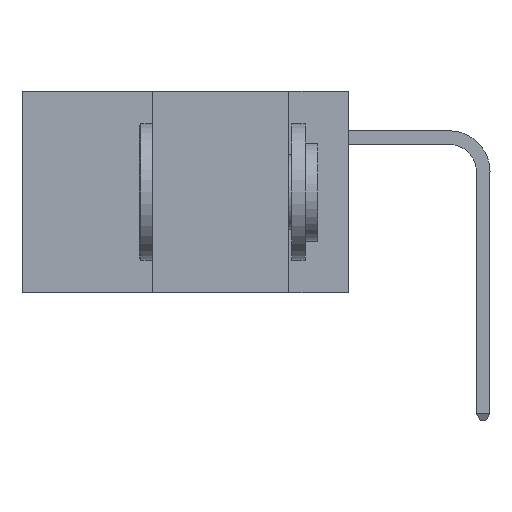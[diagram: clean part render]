
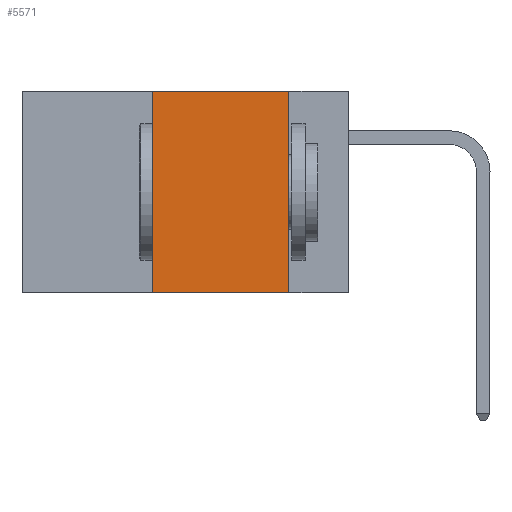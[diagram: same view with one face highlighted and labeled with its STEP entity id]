
A CAD part, left-side view. The second image highlights one B-rep face of the part: STEP entity #5571.
In plain terms, the highlighted planar face has unit normal (-1, 0, 0).
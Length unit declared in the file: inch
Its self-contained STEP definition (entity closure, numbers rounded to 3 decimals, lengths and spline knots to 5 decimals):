
#237 = CARTESIAN_POINT ( 'NONE',  ( 0., 0.36, -0.37 ) ) ;
#370 = DIRECTION ( 'NONE',  ( 0., 0., -1. ) ) ;
#1208 = AXIS2_PLACEMENT_3D ( 'NONE', #5564, #13552, #370 ) ;
#1296 = EDGE_CURVE ( 'NONE', #7038, #14603, #11462, .T. ) ;
#1375 = CARTESIAN_POINT ( 'NONE',  ( 0., 0.6, 0. ) ) ;
#2028 = LINE ( 'NONE', #10373, #7548 ) ;
#2738 = LINE ( 'NONE', #5368, #11712 ) ;
#2787 = EDGE_CURVE ( 'NONE', #7378, #13815, #3717, .T. ) ;
#3147 = EDGE_CURVE ( 'NONE', #13815, #14603, #2028, .T. ) ;
#3717 = LINE ( 'NONE', #1375, #15862 ) ;
#4545 = FACE_OUTER_BOUND ( 'NONE', #15443, .T. ) ;
#4963 = ORIENTED_EDGE ( 'NONE', *, *, #7336, .F. ) ;
#5248 = DIRECTION ( 'NONE',  ( 0., 0., 1. ) ) ;
#5305 = CARTESIAN_POINT ( 'NONE',  ( 0., 0.36, 0. ) ) ;
#5368 = CARTESIAN_POINT ( 'NONE',  ( 0., 0.36, 0. ) ) ;
#5564 = CARTESIAN_POINT ( 'NONE',  ( 0., 0.6, 0. ) ) ;
#5571 = ADVANCED_FACE ( 'NONE', ( #4545 ), #14821, .F. ) ;
#5902 = CARTESIAN_POINT ( 'NONE',  ( 0., 0.11, 0. ) ) ;
#6751 = ORIENTED_EDGE ( 'NONE', *, *, #2787, .F. ) ;
#6968 = VECTOR ( 'NONE', #13485, 39.37008 ) ;
#7038 = VERTEX_POINT ( 'NONE', #237 ) ;
#7336 = EDGE_CURVE ( 'NONE', #7038, #7378, #2738, .T. ) ;
#7378 = VERTEX_POINT ( 'NONE', #5305 ) ;
#7548 = VECTOR ( 'NONE', #9056, 39.37008 ) ;
#8417 = ORIENTED_EDGE ( 'NONE', *, *, #1296, .T. ) ;
#9056 = DIRECTION ( 'NONE',  ( 0., 0., -1. ) ) ;
#9144 = CARTESIAN_POINT ( 'NONE',  ( 0., 0.11, -0.37 ) ) ;
#10373 = CARTESIAN_POINT ( 'NONE',  ( 0., 0.11, 0. ) ) ;
#11462 = LINE ( 'NONE', #11972, #6968 ) ;
#11712 = VECTOR ( 'NONE', #5248, 39.37008 ) ;
#11972 = CARTESIAN_POINT ( 'NONE',  ( 0., 0.6, -0.37 ) ) ;
#12247 = DIRECTION ( 'NONE',  ( 0., -1., 0. ) ) ;
#13485 = DIRECTION ( 'NONE',  ( 0., -1., 0. ) ) ;
#13552 = DIRECTION ( 'NONE',  ( 1., 0., 0. ) ) ;
#13815 = VERTEX_POINT ( 'NONE', #5902 ) ;
#14603 = VERTEX_POINT ( 'NONE', #9144 ) ;
#14821 = PLANE ( 'NONE',  #1208 ) ;
#14843 = ORIENTED_EDGE ( 'NONE', *, *, #3147, .F. ) ;
#15443 = EDGE_LOOP ( 'NONE', ( #14843, #6751, #4963, #8417 ) ) ;
#15862 = VECTOR ( 'NONE', #12247, 39.37008 ) ;
